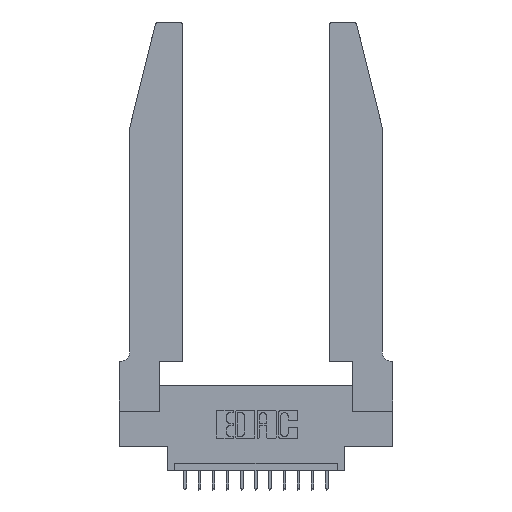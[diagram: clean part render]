
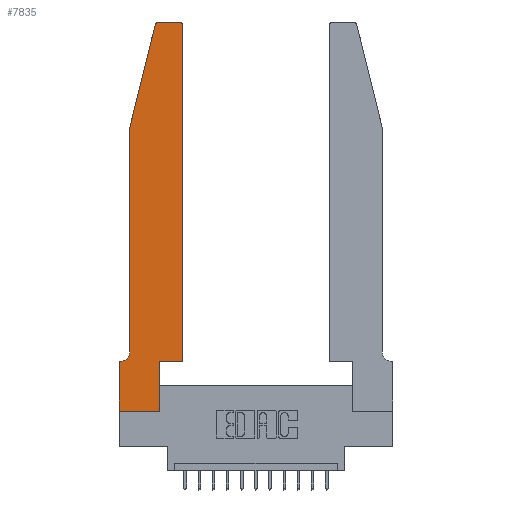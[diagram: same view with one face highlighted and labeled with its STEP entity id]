
A CAD part, top view. The second image highlights one B-rep face of the part: STEP entity #7835.
In plain terms, the highlighted planar face has unit normal (0, 0, 1).
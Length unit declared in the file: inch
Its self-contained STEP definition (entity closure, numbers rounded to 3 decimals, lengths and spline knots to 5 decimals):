
#58 = CARTESIAN_POINT ( 'NONE',  ( 0., 0., 0.37 ) ) ;
#163 = CARTESIAN_POINT ( 'NONE',  ( 0.0755, 0.35, 0.37 ) ) ;
#255 = ORIENTED_EDGE ( 'NONE', *, *, #4334, .T. ) ;
#270 = CARTESIAN_POINT ( 'NONE',  ( 0.4505, 0.35, 0.37 ) ) ;
#1516 = VERTEX_POINT ( 'NONE', #15610 ) ;
#1573 = ORIENTED_EDGE ( 'NONE', *, *, #11639, .T. ) ;
#2089 = DIRECTION ( 'NONE',  ( 0., 0., 1. ) ) ;
#2442 = VECTOR ( 'NONE', #8127, 39.37008 ) ;
#2666 = CARTESIAN_POINT ( 'NONE',  ( 0.4505, 0.35, 0.37 ) ) ;
#2736 = EDGE_CURVE ( 'NONE', #2791, #3402, #3005, .T. ) ;
#2791 = VERTEX_POINT ( 'NONE', #9957 ) ;
#2932 = DIRECTION ( 'NONE',  ( 0., -1., 0. ) ) ;
#3005 = LINE ( 'NONE', #16400, #15245 ) ;
#3402 = VERTEX_POINT ( 'NONE', #12935 ) ;
#3435 = CARTESIAN_POINT ( 'NONE',  ( 0.0755, 2., 0.37 ) ) ;
#3502 = VERTEX_POINT ( 'NONE', #12225 ) ;
#3518 = FACE_OUTER_BOUND ( 'NONE', #4270, .T. ) ;
#3827 = VECTOR ( 'NONE', #2932, 39.37008 ) ;
#4086 = CARTESIAN_POINT ( 'NONE',  ( 0.4505, 0.35, 0.37 ) ) ;
#4270 = EDGE_LOOP ( 'NONE', ( #8063, #7390, #7414, #10061, #1573, #255, #9100, #10145, #14215, #5698, #10885, #10350 ) ) ;
#4298 = DIRECTION ( 'NONE',  ( 1., 0., 0. ) ) ;
#4334 = EDGE_CURVE ( 'NONE', #3502, #10094, #17351, .T. ) ;
#4518 = VERTEX_POINT ( 'NONE', #7735 ) ;
#4949 = PLANE ( 'NONE',  #11377 ) ;
#5063 = DIRECTION ( 'NONE',  ( -1., 0., 0. ) ) ;
#5518 = VECTOR ( 'NONE', #5063, 39.37008 ) ;
#5698 = ORIENTED_EDGE ( 'NONE', *, *, #12572, .T. ) ;
#5754 = DIRECTION ( 'NONE',  ( 1., 0., 0. ) ) ;
#5904 = CARTESIAN_POINT ( 'NONE',  ( 0., 0.35, 0.37 ) ) ;
#5997 = CARTESIAN_POINT ( 'NONE',  ( 0.4205, 2.72, 0.37 ) ) ;
#6507 = CARTESIAN_POINT ( 'NONE',  ( 0.0755, 2., 0.37 ) ) ;
#6700 = CARTESIAN_POINT ( 'NONE',  ( 0.0755, 2., 0.37 ) ) ;
#6784 = EDGE_CURVE ( 'NONE', #13563, #4518, #8983, .T. ) ;
#6961 = CARTESIAN_POINT ( 'NONE',  ( 0., 0., 0.37 ) ) ;
#7390 = ORIENTED_EDGE ( 'NONE', *, *, #8421, .T. ) ;
#7414 = ORIENTED_EDGE ( 'NONE', *, *, #9688, .T. ) ;
#7683 = LINE ( 'NONE', #17097, #5518 ) ;
#7735 = CARTESIAN_POINT ( 'NONE',  ( 0.0755, 0.42, 0.37 ) ) ;
#7835 = ADVANCED_FACE ( 'NONE', ( #3518 ), #4949, .T. ) ;
#7886 = EDGE_CURVE ( 'NONE', #12939, #17253, #8985, .T. ) ;
#8063 = ORIENTED_EDGE ( 'NONE', *, *, #9017, .T. ) ;
#8127 = DIRECTION ( 'NONE',  ( 1., 0., 0. ) ) ;
#8421 = EDGE_CURVE ( 'NONE', #1516, #11455, #8871, .T. ) ;
#8871 = CIRCLE ( 'NONE', #13081, 0.03 ) ;
#8983 = LINE ( 'NONE', #6507, #9103 ) ;
#8985 = LINE ( 'NONE', #270, #17003 ) ;
#9017 = EDGE_CURVE ( 'NONE', #16576, #1516, #7683, .T. ) ;
#9062 = VECTOR ( 'NONE', #12167, 39.37008 ) ;
#9100 = ORIENTED_EDGE ( 'NONE', *, *, #11059, .T. ) ;
#9103 = VECTOR ( 'NONE', #14351, 39.37008 ) ;
#9168 = LINE ( 'NONE', #6700, #12286 ) ;
#9345 = DIRECTION ( 'NONE',  ( -0.239, -0.971, 0. ) ) ;
#9546 = LINE ( 'NONE', #13336, #3827 ) ;
#9604 = LINE ( 'NONE', #6961, #12051 ) ;
#9688 = EDGE_CURVE ( 'NONE', #11455, #13563, #9168, .T. ) ;
#9754 = CIRCLE ( 'NONE', #12006, 0.07 ) ;
#9853 = DIRECTION ( 'NONE',  ( 1., 0., 0. ) ) ;
#9957 = CARTESIAN_POINT ( 'NONE',  ( 0.2865, 0., 0.37 ) ) ;
#10030 = AXIS2_PLACEMENT_3D ( 'NONE', #5997, #14365, #10395 ) ;
#10061 = ORIENTED_EDGE ( 'NONE', *, *, #6784, .T. ) ;
#10094 = VERTEX_POINT ( 'NONE', #5904 ) ;
#10145 = ORIENTED_EDGE ( 'NONE', *, *, #16404, .T. ) ;
#10193 = DIRECTION ( 'NONE',  ( 0., 0., -1. ) ) ;
#10350 = ORIENTED_EDGE ( 'NONE', *, *, #14773, .T. ) ;
#10395 = DIRECTION ( 'NONE',  ( 1., 0., 0. ) ) ;
#10885 = ORIENTED_EDGE ( 'NONE', *, *, #7886, .T. ) ;
#10976 = CARTESIAN_POINT ( 'NONE',  ( 0.284, 2.72, 0.37 ) ) ;
#11039 = DIRECTION ( 'NONE',  ( 0., 1., 0. ) ) ;
#11059 = EDGE_CURVE ( 'NONE', #10094, #16718, #9546, .T. ) ;
#11377 = AXIS2_PLACEMENT_3D ( 'NONE', #12362, #2089, #5754 ) ;
#11455 = VERTEX_POINT ( 'NONE', #13565 ) ;
#11639 = EDGE_CURVE ( 'NONE', #4518, #3502, #9754, .T. ) ;
#12006 = AXIS2_PLACEMENT_3D ( 'NONE', #15219, #10193, #12836 ) ;
#12051 = VECTOR ( 'NONE', #9853, 39.37008 ) ;
#12167 = DIRECTION ( 'NONE',  ( -1., 0., 0. ) ) ;
#12185 = DIRECTION ( 'NONE',  ( 0., 1., 0. ) ) ;
#12225 = CARTESIAN_POINT ( 'NONE',  ( 0.0055, 0.35, 0.37 ) ) ;
#12286 = VECTOR ( 'NONE', #9345, 39.37008 ) ;
#12362 = CARTESIAN_POINT ( 'NONE',  ( 0., 0.35, 0.37 ) ) ;
#12572 = EDGE_CURVE ( 'NONE', #3402, #12939, #17363, .T. ) ;
#12836 = DIRECTION ( 'NONE',  ( -1., 0., 0. ) ) ;
#12935 = CARTESIAN_POINT ( 'NONE',  ( 0.2865, 0.35, 0.37 ) ) ;
#12939 = VERTEX_POINT ( 'NONE', #2666 ) ;
#13081 = AXIS2_PLACEMENT_3D ( 'NONE', #10976, #16344, #4298 ) ;
#13336 = CARTESIAN_POINT ( 'NONE',  ( 0., 0., 0.37 ) ) ;
#13563 = VERTEX_POINT ( 'NONE', #3435 ) ;
#13565 = CARTESIAN_POINT ( 'NONE',  ( 0.25487, 2.72718, 0.37 ) ) ;
#14215 = ORIENTED_EDGE ( 'NONE', *, *, #2736, .T. ) ;
#14351 = DIRECTION ( 'NONE',  ( 0., -1., 0. ) ) ;
#14365 = DIRECTION ( 'NONE',  ( 0., 0., 1. ) ) ;
#14773 = EDGE_CURVE ( 'NONE', #17253, #16576, #16493, .T. ) ;
#15219 = CARTESIAN_POINT ( 'NONE',  ( 0.0055, 0.42, 0.37 ) ) ;
#15245 = VECTOR ( 'NONE', #12185, 39.37008 ) ;
#15610 = CARTESIAN_POINT ( 'NONE',  ( 0.284, 2.75, 0.37 ) ) ;
#15661 = CARTESIAN_POINT ( 'NONE',  ( 0.4205, 2.75, 0.37 ) ) ;
#16344 = DIRECTION ( 'NONE',  ( 0., 0., 1. ) ) ;
#16400 = CARTESIAN_POINT ( 'NONE',  ( 0.2865, 0.35, 0.37 ) ) ;
#16404 = EDGE_CURVE ( 'NONE', #16718, #2791, #9604, .T. ) ;
#16493 = CIRCLE ( 'NONE', #10030, 0.03 ) ;
#16506 = CARTESIAN_POINT ( 'NONE',  ( 0.4505, 2.72, 0.37 ) ) ;
#16576 = VERTEX_POINT ( 'NONE', #15661 ) ;
#16718 = VERTEX_POINT ( 'NONE', #58 ) ;
#17003 = VECTOR ( 'NONE', #11039, 39.37008 ) ;
#17097 = CARTESIAN_POINT ( 'NONE',  ( 0.2605, 2.75, 0.37 ) ) ;
#17253 = VERTEX_POINT ( 'NONE', #16506 ) ;
#17351 = LINE ( 'NONE', #163, #9062 ) ;
#17363 = LINE ( 'NONE', #4086, #2442 ) ;
